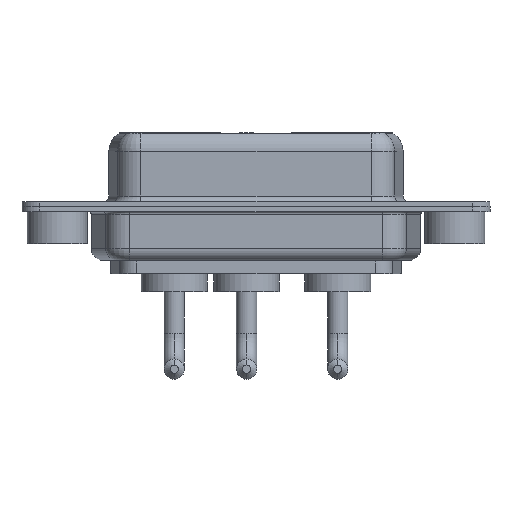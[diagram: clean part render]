
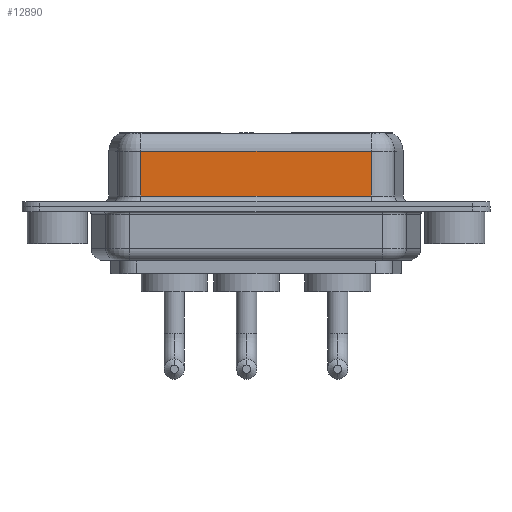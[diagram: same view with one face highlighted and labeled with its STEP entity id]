
A CAD part, front view. The second image highlights one B-rep face of the part: STEP entity #12890.
In plain terms, the highlighted planar face has unit normal (0, -1, 0).
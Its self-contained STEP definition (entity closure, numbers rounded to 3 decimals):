
#1194 = FACE_OUTER_BOUND ( 'NONE', #8448, .T. ) ;
#1497 = CARTESIAN_POINT ( 'NONE',  ( 26.287, -3.95, 0.9 ) ) ;
#1722 = CARTESIAN_POINT ( 'NONE',  ( 26.287, -3.95, 4.65 ) ) ;
#1917 = AXIS2_PLACEMENT_3D ( 'NONE', #5440, #4391, #8624 ) ;
#1929 = DIRECTION ( 'NONE',  ( 1., 0., 0. ) ) ;
#2031 = ORIENTED_EDGE ( 'NONE', *, *, #6127, .T. ) ;
#2272 = EDGE_CURVE ( 'NONE', #4288, #2929, #8044, .T. ) ;
#2299 = EDGE_CURVE ( 'NONE', #2929, #8125, #13492, .T. ) ;
#2604 = CARTESIAN_POINT ( 'NONE',  ( 7.013, -3.95, 0.9 ) ) ;
#2712 = DIRECTION ( 'NONE',  ( -1., 0., 0. ) ) ;
#2929 = VERTEX_POINT ( 'NONE', #6282 ) ;
#3354 = LINE ( 'NONE', #8769, #5284 ) ;
#3943 = LINE ( 'NONE', #11388, #10721 ) ;
#3944 = CARTESIAN_POINT ( 'NONE',  ( 7.013, -3.95, 6.4 ) ) ;
#4288 = VERTEX_POINT ( 'NONE', #4553 ) ;
#4391 = DIRECTION ( 'NONE',  ( 0., 1., 0. ) ) ;
#4553 = CARTESIAN_POINT ( 'NONE',  ( 26.287, -3.95, 4.65 ) ) ;
#5284 = VECTOR ( 'NONE', #12957, 1000. ) ;
#5440 = CARTESIAN_POINT ( 'NONE',  ( 26.287, -3.95, 6.4 ) ) ;
#6127 = EDGE_CURVE ( 'NONE', #8125, #12100, #3943, .T. ) ;
#6282 = CARTESIAN_POINT ( 'NONE',  ( 7.013, -3.95, 4.65 ) ) ;
#6482 = ORIENTED_EDGE ( 'NONE', *, *, #2272, .T. ) ;
#6799 = VECTOR ( 'NONE', #2712, 1000. ) ;
#7234 = EDGE_CURVE ( 'NONE', #4288, #12100, #3354, .T. ) ;
#7684 = ORIENTED_EDGE ( 'NONE', *, *, #2299, .T. ) ;
#8044 = LINE ( 'NONE', #1722, #6799 ) ;
#8125 = VERTEX_POINT ( 'NONE', #2604 ) ;
#8186 = DIRECTION ( 'NONE',  ( 0., 0., -1. ) ) ;
#8448 = EDGE_LOOP ( 'NONE', ( #9456, #6482, #7684, #2031 ) ) ;
#8624 = DIRECTION ( 'NONE',  ( 0., 0., 1. ) ) ;
#8695 = PLANE ( 'NONE',  #1917 ) ;
#8769 = CARTESIAN_POINT ( 'NONE',  ( 26.287, -3.95, 6.4 ) ) ;
#9456 = ORIENTED_EDGE ( 'NONE', *, *, #7234, .F. ) ;
#10721 = VECTOR ( 'NONE', #1929, 1000. ) ;
#10789 = VECTOR ( 'NONE', #8186, 1000. ) ;
#11388 = CARTESIAN_POINT ( 'NONE',  ( 26.287, -3.95, 0.9 ) ) ;
#12100 = VERTEX_POINT ( 'NONE', #1497 ) ;
#12890 = ADVANCED_FACE ( 'NONE', ( #1194 ), #8695, .F. ) ;
#12957 = DIRECTION ( 'NONE',  ( 0., 0., -1. ) ) ;
#13492 = LINE ( 'NONE', #3944, #10789 ) ;
